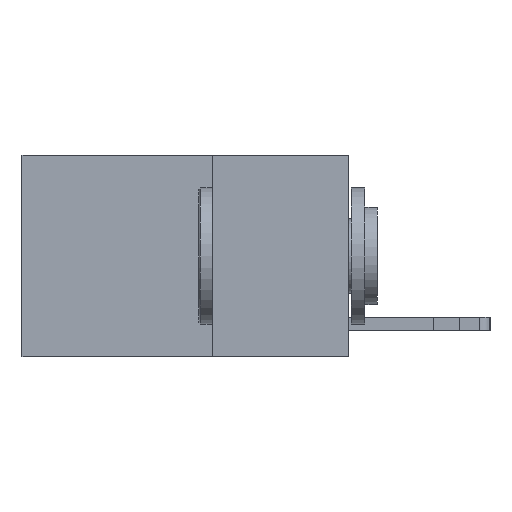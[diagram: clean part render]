
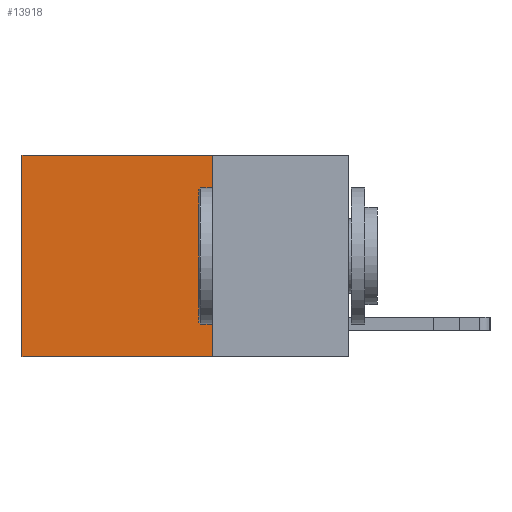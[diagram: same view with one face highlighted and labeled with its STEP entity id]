
A CAD part, left-side view. The second image highlights one B-rep face of the part: STEP entity #13918.
In plain terms, the highlighted planar face has unit normal (-1, 0, 0).
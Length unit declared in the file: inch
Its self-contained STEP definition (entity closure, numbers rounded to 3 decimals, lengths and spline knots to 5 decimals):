
#255 = EDGE_CURVE ( 'NONE', #10735, #11753, #8697, .T. ) ;
#1150 = ORIENTED_EDGE ( 'NONE', *, *, #6913, .T. ) ;
#1595 = VERTEX_POINT ( 'NONE', #11128 ) ;
#1660 = CARTESIAN_POINT ( 'NONE',  ( 0.2625, 0.25, -0.37 ) ) ;
#1663 = LINE ( 'NONE', #1741, #5209 ) ;
#1741 = CARTESIAN_POINT ( 'NONE',  ( 0.2625, 0.25, -0.37 ) ) ;
#1890 = PLANE ( 'NONE',  #14642 ) ;
#2906 = EDGE_LOOP ( 'NONE', ( #5467, #12062, #12908, #1150 ) ) ;
#3018 = LINE ( 'NONE', #15702, #6522 ) ;
#3699 = VERTEX_POINT ( 'NONE', #1660 ) ;
#4892 = EDGE_CURVE ( 'NONE', #3699, #11753, #1663, .T. ) ;
#5185 = LINE ( 'NONE', #10107, #12250 ) ;
#5209 = VECTOR ( 'NONE', #10312, 39.37008 ) ;
#5467 = ORIENTED_EDGE ( 'NONE', *, *, #255, .T. ) ;
#5760 = DIRECTION ( 'NONE',  ( 0., 0., -1. ) ) ;
#6522 = VECTOR ( 'NONE', #15369, 39.37008 ) ;
#6913 = EDGE_CURVE ( 'NONE', #1595, #10735, #3018, .T. ) ;
#7083 = CARTESIAN_POINT ( 'NONE',  ( 0.2625, 0.6, -0.37 ) ) ;
#8697 = LINE ( 'NONE', #13641, #12131 ) ;
#9141 = EDGE_CURVE ( 'NONE', #1595, #3699, #5185, .T. ) ;
#9854 = CARTESIAN_POINT ( 'NONE',  ( 0.2625, 0.6, 0. ) ) ;
#10107 = CARTESIAN_POINT ( 'NONE',  ( 0.2625, 0.25, 0. ) ) ;
#10312 = DIRECTION ( 'NONE',  ( 0., 1., 0. ) ) ;
#10735 = VERTEX_POINT ( 'NONE', #9854 ) ;
#11128 = CARTESIAN_POINT ( 'NONE',  ( 0.2625, 0.25, 0. ) ) ;
#11753 = VERTEX_POINT ( 'NONE', #7083 ) ;
#11911 = CARTESIAN_POINT ( 'NONE',  ( 0.2625, 0.25, 0. ) ) ;
#12062 = ORIENTED_EDGE ( 'NONE', *, *, #4892, .F. ) ;
#12131 = VECTOR ( 'NONE', #12427, 39.37008 ) ;
#12250 = VECTOR ( 'NONE', #13832, 39.37008 ) ;
#12427 = DIRECTION ( 'NONE',  ( 0., 0., -1. ) ) ;
#12908 = ORIENTED_EDGE ( 'NONE', *, *, #9141, .F. ) ;
#13208 = FACE_OUTER_BOUND ( 'NONE', #2906, .T. ) ;
#13641 = CARTESIAN_POINT ( 'NONE',  ( 0.2625, 0.6, 0. ) ) ;
#13832 = DIRECTION ( 'NONE',  ( 0., 0., -1. ) ) ;
#13918 = ADVANCED_FACE ( 'NONE', ( #13208 ), #1890, .F. ) ;
#14098 = DIRECTION ( 'NONE',  ( 1., 0., 0. ) ) ;
#14642 = AXIS2_PLACEMENT_3D ( 'NONE', #11911, #14098, #5760 ) ;
#15369 = DIRECTION ( 'NONE',  ( 0., 1., 0. ) ) ;
#15702 = CARTESIAN_POINT ( 'NONE',  ( 0.2625, 0.25, 0. ) ) ;
